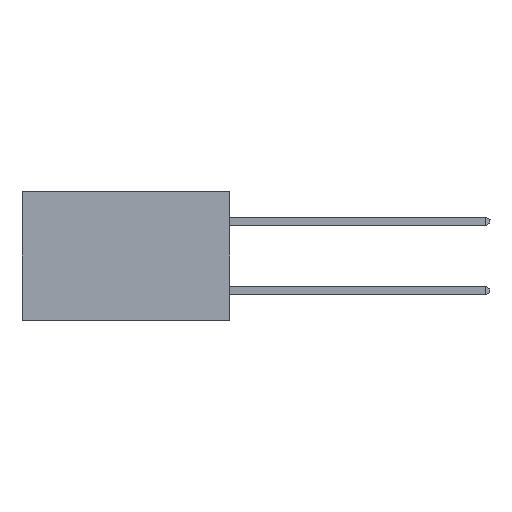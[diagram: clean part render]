
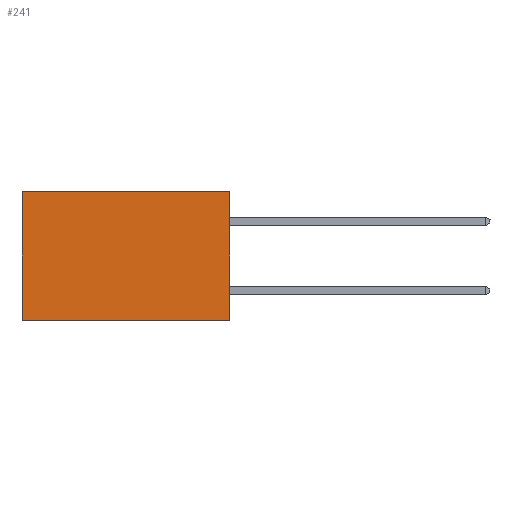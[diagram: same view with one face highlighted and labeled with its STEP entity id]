
A CAD part, left-side view. The second image highlights one B-rep face of the part: STEP entity #241.
In plain terms, the highlighted planar face has unit normal (-1, 0, 0).
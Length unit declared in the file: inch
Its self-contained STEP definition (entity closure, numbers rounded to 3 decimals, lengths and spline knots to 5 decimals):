
#241 = ADVANCED_FACE ( 'NONE', ( #6810 ), #1350, .F. ) ;
#918 = LINE ( 'NONE', #16109, #21422 ) ;
#1023 = VECTOR ( 'NONE', #6157, 39.37008 ) ;
#1350 = PLANE ( 'NONE',  #8293 ) ;
#2028 = VERTEX_POINT ( 'NONE', #17358 ) ;
#2390 = ORIENTED_EDGE ( 'NONE', *, *, #3398, .T. ) ;
#2864 = EDGE_CURVE ( 'NONE', #15945, #2028, #20033, .T. ) ;
#3244 = CARTESIAN_POINT ( 'NONE',  ( 0.298, 0., 0. ) ) ;
#3398 = EDGE_CURVE ( 'NONE', #15945, #5774, #13541, .T. ) ;
#4273 = VERTEX_POINT ( 'NONE', #15284 ) ;
#4962 = DIRECTION ( 'NONE',  ( 0., 0., -1. ) ) ;
#5774 = VERTEX_POINT ( 'NONE', #8387 ) ;
#6157 = DIRECTION ( 'NONE',  ( 0., 1., 0. ) ) ;
#6810 = FACE_OUTER_BOUND ( 'NONE', #15648, .T. ) ;
#8293 = AXIS2_PLACEMENT_3D ( 'NONE', #3244, #10540, #4962 ) ;
#8387 = CARTESIAN_POINT ( 'NONE',  ( 0.298, 0.6, 0. ) ) ;
#10540 = DIRECTION ( 'NONE',  ( 1., 0., 0. ) ) ;
#11377 = EDGE_CURVE ( 'NONE', #2028, #4273, #16463, .T. ) ;
#11401 = DIRECTION ( 'NONE',  ( 0., 0., -1. ) ) ;
#13400 = CARTESIAN_POINT ( 'NONE',  ( 0.298, 0., 0. ) ) ;
#13541 = LINE ( 'NONE', #22318, #20279 ) ;
#13744 = ORIENTED_EDGE ( 'NONE', *, *, #2864, .F. ) ;
#14131 = VECTOR ( 'NONE', #11401, 39.37008 ) ;
#14379 = DIRECTION ( 'NONE',  ( 0., 0., -1. ) ) ;
#15284 = CARTESIAN_POINT ( 'NONE',  ( 0.298, 0.6, -0.37 ) ) ;
#15435 = EDGE_CURVE ( 'NONE', #5774, #4273, #918, .T. ) ;
#15587 = CARTESIAN_POINT ( 'NONE',  ( 0.298, 0., 0. ) ) ;
#15648 = EDGE_LOOP ( 'NONE', ( #23170, #16936, #13744, #2390 ) ) ;
#15945 = VERTEX_POINT ( 'NONE', #13400 ) ;
#16109 = CARTESIAN_POINT ( 'NONE',  ( 0.298, 0.6, 0. ) ) ;
#16463 = LINE ( 'NONE', #20366, #1023 ) ;
#16936 = ORIENTED_EDGE ( 'NONE', *, *, #11377, .F. ) ;
#17358 = CARTESIAN_POINT ( 'NONE',  ( 0.298, 0., -0.37 ) ) ;
#20033 = LINE ( 'NONE', #15587, #14131 ) ;
#20279 = VECTOR ( 'NONE', #20549, 39.37008 ) ;
#20366 = CARTESIAN_POINT ( 'NONE',  ( 0.298, 0., -0.37 ) ) ;
#20549 = DIRECTION ( 'NONE',  ( 0., 1., 0. ) ) ;
#21422 = VECTOR ( 'NONE', #14379, 39.37008 ) ;
#22318 = CARTESIAN_POINT ( 'NONE',  ( 0.298, 0., 0. ) ) ;
#23170 = ORIENTED_EDGE ( 'NONE', *, *, #15435, .T. ) ;
